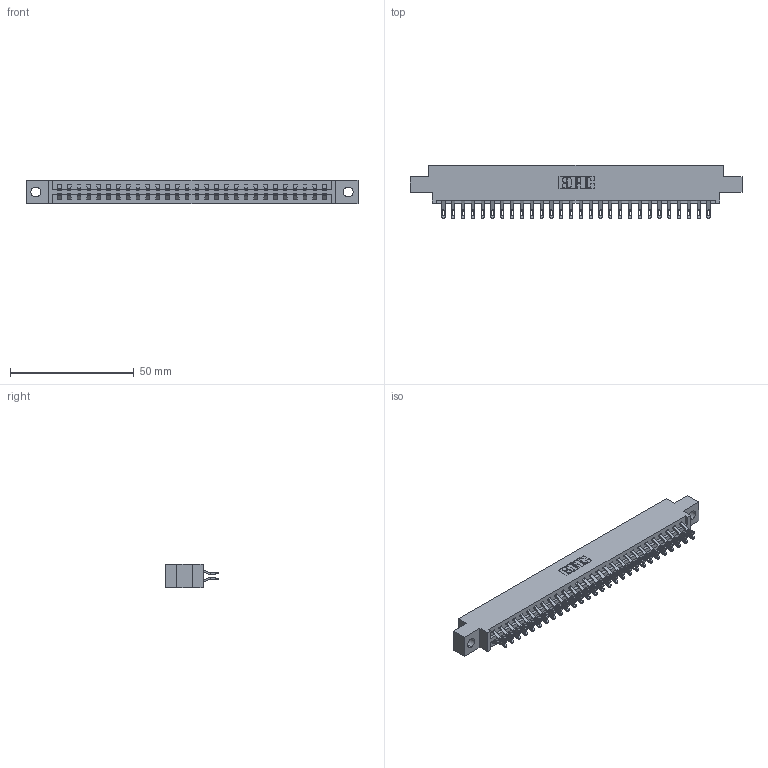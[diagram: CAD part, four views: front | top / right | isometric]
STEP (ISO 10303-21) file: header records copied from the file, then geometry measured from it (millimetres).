
FILE_DESCRIPTION (( 'STEP AP203' ), '1' );
FILE_NAME ('387-056-555-804.STEP', '2018-09-21T00:15:58', ( '' ), ( '' ), 'SwSTEP 2.0', 'SolidWorks 2016', '' );
FILE_SCHEMA (( 'CONFIG_CONTROL_DESIGN' ));
Length unit declared in the file: inch
Products named in the file (3): 345-292-001_555 Tail; 387-056-555-804; 337 Part_0.170 Offset - 0.156 Dia-TH
Assembly tree (57 placements, depth 2):
  387-056-555-804
    337 Part_0.170 Offset - 0.156 Dia-TH
    345-292-001_555 Tail  x56
Bounding box: 133.96 x 21.47 x 9.4 mm (x, y, z)
Volume: 13888.4 mm3; surface area: 16082.3 mm2
Topology: 57 solids, 57 shells, 3478 faces, 10907 edges, 7270 vertices
Faces by surface type: plane 2090, cylinder 1388
Entity records: 23981 total; most frequent: CARTESIAN_POINT 4088, ORIENTED_EDGE 3994, DIRECTION 3473, EDGE_CURVE 1997, LINE 1849, VECTOR 1849, VERTEX_POINT 1330, AXIS2_PLACEMENT_3D 812
